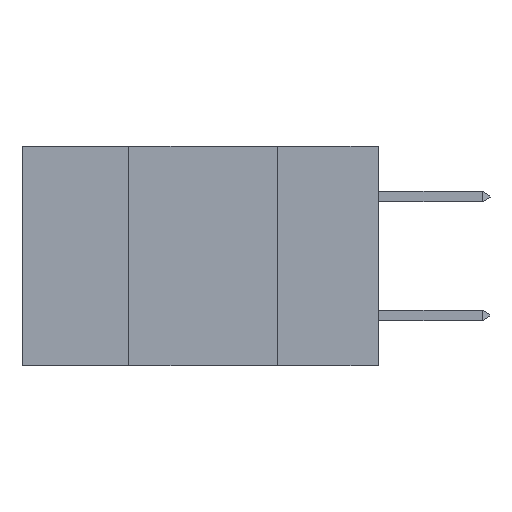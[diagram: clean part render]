
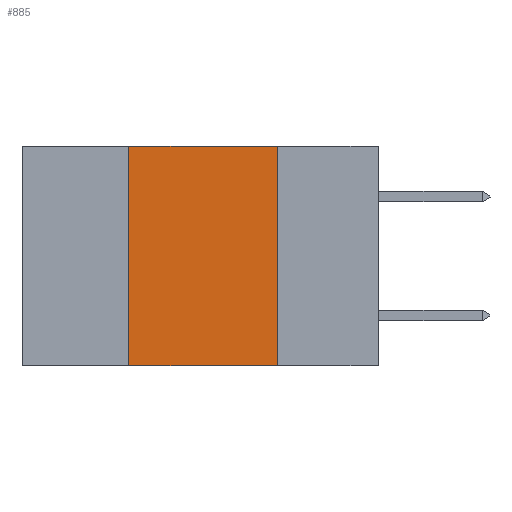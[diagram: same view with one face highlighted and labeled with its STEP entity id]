
A CAD part, left-side view. The second image highlights one B-rep face of the part: STEP entity #885.
In plain terms, the highlighted planar face has unit normal (-1, 0, 0).
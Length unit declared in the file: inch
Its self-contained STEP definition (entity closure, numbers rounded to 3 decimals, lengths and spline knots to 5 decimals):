
#842 = EDGE_CURVE ( 'NONE', #26225, #13435, #13856, .T. ) ;
#859 = VECTOR ( 'NONE', #5512, 39.37008 ) ;
#885 = ADVANCED_FACE ( 'NONE', ( #2571 ), #13935, .F. ) ;
#2347 = CARTESIAN_POINT ( 'NONE',  ( 0., 0.42, 0. ) ) ;
#2571 = FACE_OUTER_BOUND ( 'NONE', #5968, .T. ) ;
#2587 = CARTESIAN_POINT ( 'NONE',  ( 0., 0.42, -0.37 ) ) ;
#3539 = CARTESIAN_POINT ( 'NONE',  ( 0., 0.17, 0. ) ) ;
#5512 = DIRECTION ( 'NONE',  ( 0., -1., 0. ) ) ;
#5968 = EDGE_LOOP ( 'NONE', ( #19846, #9287, #10598, #23155 ) ) ;
#6234 = EDGE_CURVE ( 'NONE', #13435, #20151, #19980, .T. ) ;
#8071 = CARTESIAN_POINT ( 'NONE',  ( 0., 0.6, 0. ) ) ;
#8246 = VECTOR ( 'NONE', #25672, 39.37008 ) ;
#9287 = ORIENTED_EDGE ( 'NONE', *, *, #6234, .F. ) ;
#9435 = AXIS2_PLACEMENT_3D ( 'NONE', #25175, #24269, #24977 ) ;
#10598 = ORIENTED_EDGE ( 'NONE', *, *, #842, .F. ) ;
#13435 = VERTEX_POINT ( 'NONE', #2347 ) ;
#13856 = LINE ( 'NONE', #2587, #8246 ) ;
#13935 = PLANE ( 'NONE',  #9435 ) ;
#14337 = VECTOR ( 'NONE', #18677, 39.37008 ) ;
#14875 = CARTESIAN_POINT ( 'NONE',  ( 0., 0.17, -0.37 ) ) ;
#14970 = CARTESIAN_POINT ( 'NONE',  ( 0., 0.17, -0.37 ) ) ;
#15641 = EDGE_CURVE ( 'NONE', #26225, #25823, #17839, .T. ) ;
#17004 = DIRECTION ( 'NONE',  ( 0., 0., -1. ) ) ;
#17839 = LINE ( 'NONE', #26465, #859 ) ;
#18677 = DIRECTION ( 'NONE',  ( 0., -1., 0. ) ) ;
#19846 = ORIENTED_EDGE ( 'NONE', *, *, #25786, .F. ) ;
#19980 = LINE ( 'NONE', #8071, #14337 ) ;
#20151 = VERTEX_POINT ( 'NONE', #3539 ) ;
#20525 = CARTESIAN_POINT ( 'NONE',  ( 0., 0.42, -0.37 ) ) ;
#22192 = LINE ( 'NONE', #14875, #26960 ) ;
#23155 = ORIENTED_EDGE ( 'NONE', *, *, #15641, .T. ) ;
#24269 = DIRECTION ( 'NONE',  ( 1., 0., 0. ) ) ;
#24977 = DIRECTION ( 'NONE',  ( 0., 0., -1. ) ) ;
#25175 = CARTESIAN_POINT ( 'NONE',  ( 0., 0.6, 0. ) ) ;
#25672 = DIRECTION ( 'NONE',  ( 0., 0., 1. ) ) ;
#25786 = EDGE_CURVE ( 'NONE', #20151, #25823, #22192, .T. ) ;
#25823 = VERTEX_POINT ( 'NONE', #14970 ) ;
#26225 = VERTEX_POINT ( 'NONE', #20525 ) ;
#26465 = CARTESIAN_POINT ( 'NONE',  ( 0., 0.6, -0.37 ) ) ;
#26960 = VECTOR ( 'NONE', #17004, 39.37008 ) ;
